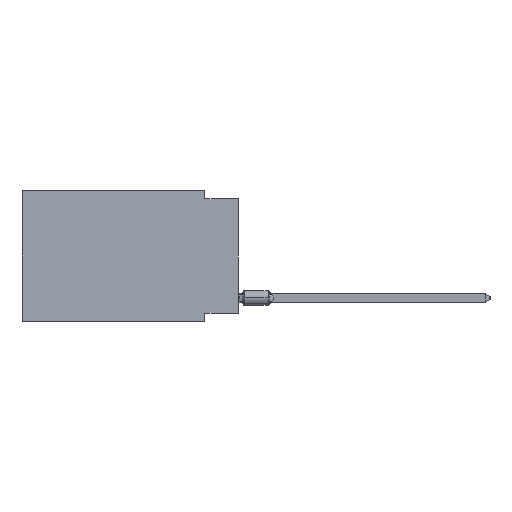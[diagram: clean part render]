
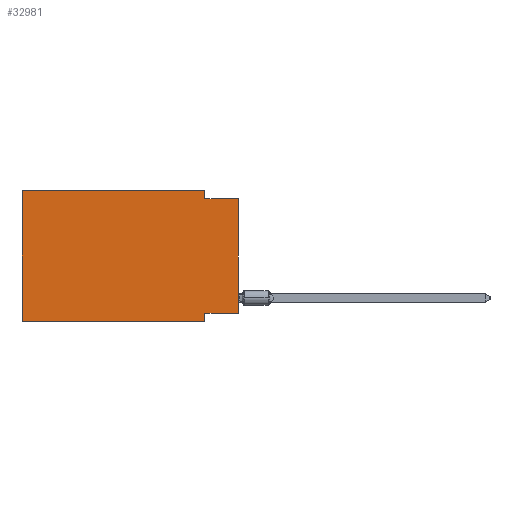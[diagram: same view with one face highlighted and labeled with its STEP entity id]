
A CAD part, left-side view. The second image highlights one B-rep face of the part: STEP entity #32981.
In plain terms, the highlighted planar face has unit normal (-1, 0, 0).
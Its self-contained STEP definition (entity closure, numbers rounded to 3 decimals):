
#2470 = VECTOR ( 'NONE', #26979, 1000. ) ;
#2563 = DIRECTION ( 'NONE',  ( 0., -1., 0. ) ) ;
#3202 = CARTESIAN_POINT ( 'NONE',  ( 0., 16.383, -9.906 ) ) ;
#3776 = VECTOR ( 'NONE', #6490, 1000. ) ;
#4923 = VERTEX_POINT ( 'NONE', #10126 ) ;
#6217 = CARTESIAN_POINT ( 'NONE',  ( 0., 16.383, -9.906 ) ) ;
#6490 = DIRECTION ( 'NONE',  ( 0., 0., 1. ) ) ;
#7590 = LINE ( 'NONE', #3202, #24930 ) ;
#9572 = VERTEX_POINT ( 'NONE', #21719 ) ;
#10126 = CARTESIAN_POINT ( 'NONE',  ( 0., 2.54, 0. ) ) ;
#10621 = LINE ( 'NONE', #16630, #2470 ) ;
#10853 = DIRECTION ( 'NONE',  ( 0., 0., -1. ) ) ;
#11635 = DIRECTION ( 'NONE',  ( 1., 0., 0. ) ) ;
#13437 = CARTESIAN_POINT ( 'NONE',  ( 0., 0., -9.271 ) ) ;
#13694 = ORIENTED_EDGE ( 'NONE', *, *, #43718, .F. ) ;
#16373 = ORIENTED_EDGE ( 'NONE', *, *, #23765, .F. ) ;
#16630 = CARTESIAN_POINT ( 'NONE',  ( 0., 0., -0.635 ) ) ;
#16657 = PLANE ( 'NONE',  #39383 ) ;
#16857 = LINE ( 'NONE', #22859, #3776 ) ;
#19716 = LINE ( 'NONE', #40128, #29797 ) ;
#19988 = EDGE_CURVE ( 'NONE', #58300, #39636, #19716, .T. ) ;
#20309 = CARTESIAN_POINT ( 'NONE',  ( 0., 0., -0.635 ) ) ;
#21719 = CARTESIAN_POINT ( 'NONE',  ( 0., 2.54, -0.635 ) ) ;
#22859 = CARTESIAN_POINT ( 'NONE',  ( 0., 16.383, 0. ) ) ;
#23146 = CARTESIAN_POINT ( 'NONE',  ( 0., 2.54, -9.906 ) ) ;
#23464 = DIRECTION ( 'NONE',  ( 0., 1., 0. ) ) ;
#23765 = EDGE_CURVE ( 'NONE', #58300, #42893, #50222, .T. ) ;
#24930 = VECTOR ( 'NONE', #2563, 1000. ) ;
#25387 = ORIENTED_EDGE ( 'NONE', *, *, #65524, .F. ) ;
#26949 = VECTOR ( 'NONE', #23464, 1000. ) ;
#26979 = DIRECTION ( 'NONE',  ( 0., -1., 0. ) ) ;
#28063 = VERTEX_POINT ( 'NONE', #23146 ) ;
#28573 = DIRECTION ( 'NONE',  ( 0., -1., 0. ) ) ;
#29797 = VECTOR ( 'NONE', #60569, 1000. ) ;
#31450 = LINE ( 'NONE', #46510, #53637 ) ;
#32038 = DIRECTION ( 'NONE',  ( 0., 0., -1. ) ) ;
#32981 = ADVANCED_FACE ( 'NONE', ( #62530 ), #16657, .F. ) ;
#36261 = EDGE_CURVE ( 'NONE', #42893, #28063, #31450, .T. ) ;
#36587 = CARTESIAN_POINT ( 'NONE',  ( 0., 2.54, 0. ) ) ;
#36631 = ORIENTED_EDGE ( 'NONE', *, *, #36261, .F. ) ;
#37050 = CARTESIAN_POINT ( 'NONE',  ( 0., 16.383, 0. ) ) ;
#39383 = AXIS2_PLACEMENT_3D ( 'NONE', #37050, #11635, #32038 ) ;
#39636 = VERTEX_POINT ( 'NONE', #20309 ) ;
#39720 = EDGE_CURVE ( 'NONE', #9572, #39636, #10621, .T. ) ;
#40128 = CARTESIAN_POINT ( 'NONE',  ( 0., 0., 0. ) ) ;
#40846 = VECTOR ( 'NONE', #10853, 1000. ) ;
#41798 = EDGE_CURVE ( 'NONE', #49828, #28063, #7590, .T. ) ;
#42488 = ORIENTED_EDGE ( 'NONE', *, *, #39720, .F. ) ;
#42893 = VERTEX_POINT ( 'NONE', #45839 ) ;
#43012 = ORIENTED_EDGE ( 'NONE', *, *, #19988, .T. ) ;
#43718 = EDGE_CURVE ( 'NONE', #49828, #64661, #16857, .T. ) ;
#45839 = CARTESIAN_POINT ( 'NONE',  ( 0., 2.54, -9.271 ) ) ;
#46510 = CARTESIAN_POINT ( 'NONE',  ( 0., 2.54, -9.906 ) ) ;
#47454 = ORIENTED_EDGE ( 'NONE', *, *, #41798, .T. ) ;
#49656 = CARTESIAN_POINT ( 'NONE',  ( 0., 16.383, 0. ) ) ;
#49828 = VERTEX_POINT ( 'NONE', #6217 ) ;
#50222 = LINE ( 'NONE', #13437, #26949 ) ;
#51118 = EDGE_LOOP ( 'NONE', ( #43012, #42488, #25387, #63604, #13694, #47454, #36631, #16373 ) ) ;
#53637 = VECTOR ( 'NONE', #61259, 1000. ) ;
#55329 = EDGE_CURVE ( 'NONE', #64661, #4923, #65087, .T. ) ;
#57606 = CARTESIAN_POINT ( 'NONE',  ( 0., 0., -9.271 ) ) ;
#58300 = VERTEX_POINT ( 'NONE', #57606 ) ;
#59158 = VECTOR ( 'NONE', #28573, 1000. ) ;
#60569 = DIRECTION ( 'NONE',  ( 0., 0., 1. ) ) ;
#61259 = DIRECTION ( 'NONE',  ( 0., 0., -1. ) ) ;
#61300 = CARTESIAN_POINT ( 'NONE',  ( 0., 16.383, 0. ) ) ;
#61390 = LINE ( 'NONE', #36587, #40846 ) ;
#62530 = FACE_OUTER_BOUND ( 'NONE', #51118, .T. ) ;
#63604 = ORIENTED_EDGE ( 'NONE', *, *, #55329, .F. ) ;
#64661 = VERTEX_POINT ( 'NONE', #61300 ) ;
#65087 = LINE ( 'NONE', #49656, #59158 ) ;
#65524 = EDGE_CURVE ( 'NONE', #4923, #9572, #61390, .T. ) ;
